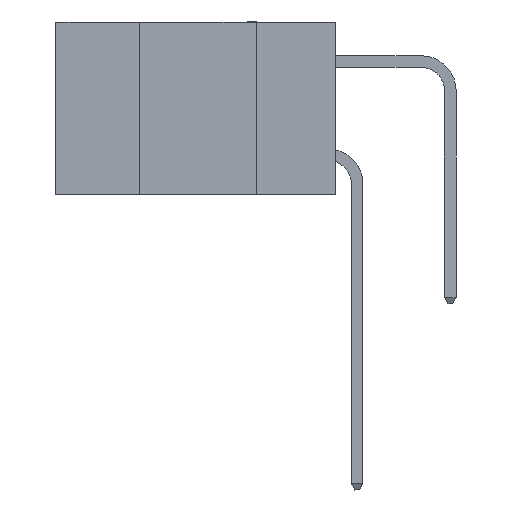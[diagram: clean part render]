
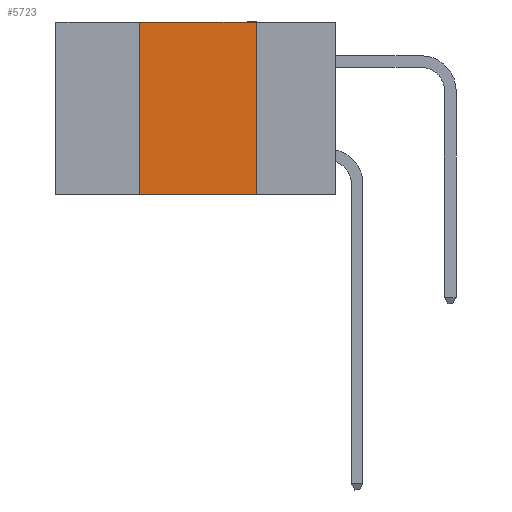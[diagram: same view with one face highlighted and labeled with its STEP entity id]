
A CAD part, left-side view. The second image highlights one B-rep face of the part: STEP entity #5723.
In plain terms, the highlighted planar face has unit normal (-1, 0, 0).
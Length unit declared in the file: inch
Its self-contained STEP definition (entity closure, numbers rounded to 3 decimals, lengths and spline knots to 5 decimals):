
#368 = VECTOR ( 'NONE', #2682, 39.37008 ) ;
#999 = DIRECTION ( 'NONE',  ( 0., -1., 0. ) ) ;
#1896 = VERTEX_POINT ( 'NONE', #35908 ) ;
#2037 = VERTEX_POINT ( 'NONE', #12457 ) ;
#2682 = DIRECTION ( 'NONE',  ( 0., 0., 1. ) ) ;
#2869 = AXIS2_PLACEMENT_3D ( 'NONE', #4580, #7246, #28398 ) ;
#3068 = CARTESIAN_POINT ( 'NONE',  ( 0., 0.6, -0.37 ) ) ;
#3538 = EDGE_CURVE ( 'NONE', #10266, #27273, #15644, .T. ) ;
#3837 = VECTOR ( 'NONE', #999, 39.37008 ) ;
#4580 = CARTESIAN_POINT ( 'NONE',  ( 0., 0.6, 0. ) ) ;
#5723 = ADVANCED_FACE ( 'NONE', ( #24535 ), #22494, .F. ) ;
#5747 = LINE ( 'NONE', #28420, #3837 ) ;
#7246 = DIRECTION ( 'NONE',  ( 1., 0., 0. ) ) ;
#7920 = CARTESIAN_POINT ( 'NONE',  ( 0., 0.42, -0.37 ) ) ;
#8271 = VECTOR ( 'NONE', #27555, 39.37008 ) ;
#8573 = CARTESIAN_POINT ( 'NONE',  ( 0., 0.42, 0. ) ) ;
#10266 = VERTEX_POINT ( 'NONE', #7920 ) ;
#12194 = ORIENTED_EDGE ( 'NONE', *, *, #20894, .T. ) ;
#12457 = CARTESIAN_POINT ( 'NONE',  ( 0., 0.17, 0. ) ) ;
#13976 = DIRECTION ( 'NONE',  ( 0., 0., -1. ) ) ;
#15644 = LINE ( 'NONE', #8573, #368 ) ;
#20894 = EDGE_CURVE ( 'NONE', #10266, #1896, #24758, .T. ) ;
#22494 = PLANE ( 'NONE',  #2869 ) ;
#22565 = EDGE_CURVE ( 'NONE', #27273, #2037, #5747, .T. ) ;
#22772 = EDGE_LOOP ( 'NONE', ( #26641, #32084, #30737, #12194 ) ) ;
#24535 = FACE_OUTER_BOUND ( 'NONE', #22772, .T. ) ;
#24758 = LINE ( 'NONE', #3068, #8271 ) ;
#26641 = ORIENTED_EDGE ( 'NONE', *, *, #31021, .F. ) ;
#27273 = VERTEX_POINT ( 'NONE', #32021 ) ;
#27555 = DIRECTION ( 'NONE',  ( 0., -1., 0. ) ) ;
#28398 = DIRECTION ( 'NONE',  ( 0., 0., -1. ) ) ;
#28420 = CARTESIAN_POINT ( 'NONE',  ( 0., 0.6, 0. ) ) ;
#30737 = ORIENTED_EDGE ( 'NONE', *, *, #3538, .F. ) ;
#31021 = EDGE_CURVE ( 'NONE', #2037, #1896, #31939, .T. ) ;
#31939 = LINE ( 'NONE', #32040, #33330 ) ;
#32021 = CARTESIAN_POINT ( 'NONE',  ( 0., 0.42, 0. ) ) ;
#32040 = CARTESIAN_POINT ( 'NONE',  ( 0., 0.17, 0. ) ) ;
#32084 = ORIENTED_EDGE ( 'NONE', *, *, #22565, .F. ) ;
#33330 = VECTOR ( 'NONE', #13976, 39.37008 ) ;
#35908 = CARTESIAN_POINT ( 'NONE',  ( 0., 0.17, -0.37 ) ) ;
